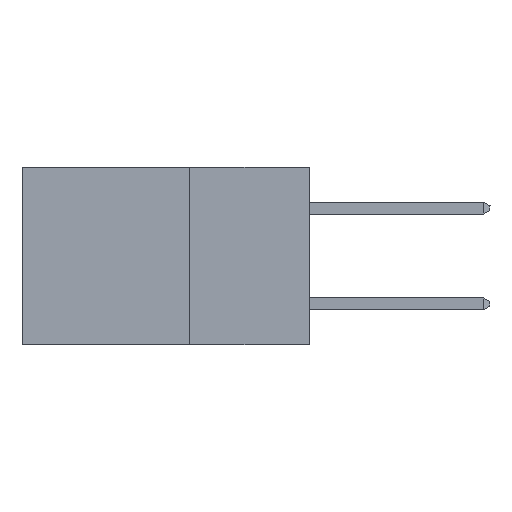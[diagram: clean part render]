
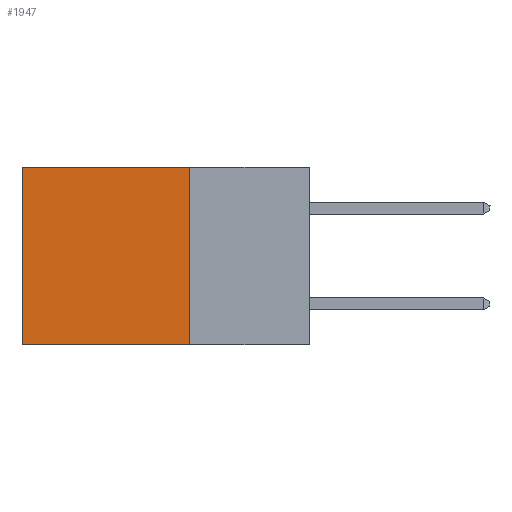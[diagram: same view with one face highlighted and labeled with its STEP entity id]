
A CAD part, left-side view. The second image highlights one B-rep face of the part: STEP entity #1947.
In plain terms, the highlighted planar face has unit normal (-1, 0, 0).
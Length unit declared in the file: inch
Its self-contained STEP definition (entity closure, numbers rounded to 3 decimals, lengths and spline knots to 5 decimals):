
#1447 = VECTOR ( 'NONE', #11017, 39.37008 ) ;
#1493 = VERTEX_POINT ( 'NONE', #9271 ) ;
#1637 = CARTESIAN_POINT ( 'NONE',  ( 0.2875, 0.25, 0. ) ) ;
#1947 = ADVANCED_FACE ( 'NONE', ( #9395 ), #4751, .F. ) ;
#2408 = DIRECTION ( 'NONE',  ( 0., 1., 0. ) ) ;
#2544 = DIRECTION ( 'NONE',  ( 0., 0., -1. ) ) ;
#2983 = VECTOR ( 'NONE', #15316, 39.37008 ) ;
#4751 = PLANE ( 'NONE',  #17094 ) ;
#5161 = CARTESIAN_POINT ( 'NONE',  ( 0.2875, 0.25, 0. ) ) ;
#6421 = VECTOR ( 'NONE', #2408, 39.37008 ) ;
#6845 = ORIENTED_EDGE ( 'NONE', *, *, #15579, .T. ) ;
#6943 = CARTESIAN_POINT ( 'NONE',  ( 0.2875, 0.6, 0. ) ) ;
#7134 = EDGE_CURVE ( 'NONE', #1493, #10057, #14877, .T. ) ;
#8163 = LINE ( 'NONE', #9755, #2983 ) ;
#8398 = ORIENTED_EDGE ( 'NONE', *, *, #7134, .F. ) ;
#8403 = CARTESIAN_POINT ( 'NONE',  ( 0.2875, 0.25, 0. ) ) ;
#8758 = EDGE_CURVE ( 'NONE', #12994, #1493, #15672, .T. ) ;
#9271 = CARTESIAN_POINT ( 'NONE',  ( 0.2875, 0.25, -0.37 ) ) ;
#9395 = FACE_OUTER_BOUND ( 'NONE', #10281, .T. ) ;
#9755 = CARTESIAN_POINT ( 'NONE',  ( 0.2875, 0.25, 0. ) ) ;
#10057 = VERTEX_POINT ( 'NONE', #16087 ) ;
#10281 = EDGE_LOOP ( 'NONE', ( #11315, #8398, #17931, #6845 ) ) ;
#10822 = DIRECTION ( 'NONE',  ( 1., 0., 0. ) ) ;
#11017 = DIRECTION ( 'NONE',  ( 0., 0., -1. ) ) ;
#11315 = ORIENTED_EDGE ( 'NONE', *, *, #13507, .T. ) ;
#11388 = DIRECTION ( 'NONE',  ( 0., 0., -1. ) ) ;
#12285 = CARTESIAN_POINT ( 'NONE',  ( 0.2875, 0.6, 0. ) ) ;
#12994 = VERTEX_POINT ( 'NONE', #8403 ) ;
#13507 = EDGE_CURVE ( 'NONE', #14272, #10057, #15943, .T. ) ;
#14272 = VERTEX_POINT ( 'NONE', #12285 ) ;
#14589 = VECTOR ( 'NONE', #11388, 39.37008 ) ;
#14877 = LINE ( 'NONE', #14916, #6421 ) ;
#14916 = CARTESIAN_POINT ( 'NONE',  ( 0.2875, 0.25, -0.37 ) ) ;
#15316 = DIRECTION ( 'NONE',  ( 0., 1., 0. ) ) ;
#15579 = EDGE_CURVE ( 'NONE', #12994, #14272, #8163, .T. ) ;
#15672 = LINE ( 'NONE', #1637, #14589 ) ;
#15943 = LINE ( 'NONE', #6943, #1447 ) ;
#16087 = CARTESIAN_POINT ( 'NONE',  ( 0.2875, 0.6, -0.37 ) ) ;
#17094 = AXIS2_PLACEMENT_3D ( 'NONE', #5161, #10822, #2544 ) ;
#17931 = ORIENTED_EDGE ( 'NONE', *, *, #8758, .F. ) ;
